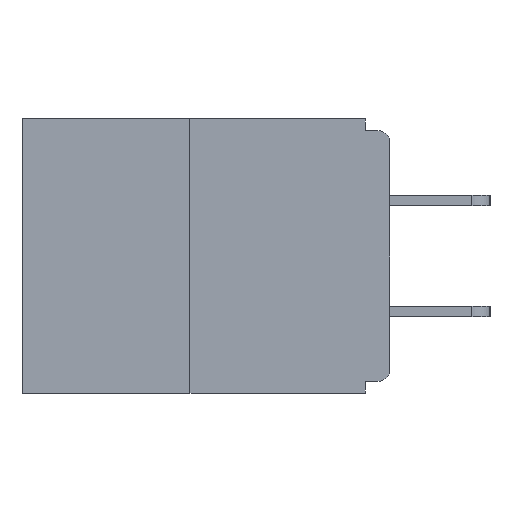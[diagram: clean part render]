
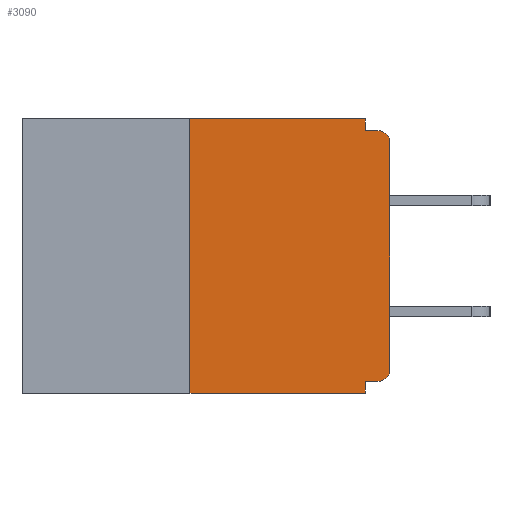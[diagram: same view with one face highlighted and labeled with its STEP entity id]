
A CAD part, left-side view. The second image highlights one B-rep face of the part: STEP entity #3090.
In plain terms, the highlighted planar face has unit normal (-1, 0, 0).
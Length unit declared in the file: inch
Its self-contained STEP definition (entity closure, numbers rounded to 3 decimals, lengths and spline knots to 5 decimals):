
#253 = DIRECTION ( 'NONE',  ( 0., 0., -1. ) ) ;
#407 = EDGE_LOOP ( 'NONE', ( #10331, #9916, #10755, #5354, #20333, #19173, #6647, #4844, #19789, #19438 ) ) ;
#422 = CARTESIAN_POINT ( 'NONE',  ( 0., 0.25, 0. ) ) ;
#709 = AXIS2_PLACEMENT_3D ( 'NONE', #9623, #9401, #14235 ) ;
#1042 = VERTEX_POINT ( 'NONE', #7243 ) ;
#1128 = DIRECTION ( 'NONE',  ( 0., 0., -1. ) ) ;
#1490 = VERTEX_POINT ( 'NONE', #20163 ) ;
#1599 = CARTESIAN_POINT ( 'NONE',  ( 0., 0.015, -0.03 ) ) ;
#1653 = CARTESIAN_POINT ( 'NONE',  ( 0., 0.015, -0.328 ) ) ;
#1782 = DIRECTION ( 'NONE',  ( -1., 0., 0. ) ) ;
#2114 = LINE ( 'NONE', #14943, #3448 ) ;
#2615 = CARTESIAN_POINT ( 'NONE',  ( 0., 0., 0. ) ) ;
#2814 = VECTOR ( 'NONE', #1128, 39.37008 ) ;
#3090 = ADVANCED_FACE ( 'NONE', ( #9512 ), #6262, .F. ) ;
#3448 = VECTOR ( 'NONE', #12514, 39.37008 ) ;
#3585 = DIRECTION ( 'NONE',  ( -1., 0., 0. ) ) ;
#4149 = CARTESIAN_POINT ( 'NONE',  ( 0., 0.031, -0.343 ) ) ;
#4844 = ORIENTED_EDGE ( 'NONE', *, *, #12302, .T. ) ;
#5054 = VERTEX_POINT ( 'NONE', #9495 ) ;
#5354 = ORIENTED_EDGE ( 'NONE', *, *, #20335, .F. ) ;
#5478 = EDGE_CURVE ( 'NONE', #9140, #5054, #14871, .T. ) ;
#5546 = VERTEX_POINT ( 'NONE', #13493 ) ;
#6262 = PLANE ( 'NONE',  #709 ) ;
#6422 = CARTESIAN_POINT ( 'NONE',  ( 0., 0.015, -0.313 ) ) ;
#6558 = LINE ( 'NONE', #6652, #14141 ) ;
#6647 = ORIENTED_EDGE ( 'NONE', *, *, #11553, .T. ) ;
#6652 = CARTESIAN_POINT ( 'NONE',  ( 0., 0., -0.015 ) ) ;
#6838 = DIRECTION ( 'NONE',  ( 0., 0., 1. ) ) ;
#7002 = DIRECTION ( 'NONE',  ( 0., 0., -1. ) ) ;
#7243 = CARTESIAN_POINT ( 'NONE',  ( 0., 0.031, -0.343 ) ) ;
#7354 = EDGE_CURVE ( 'NONE', #11797, #17008, #15986, .T. ) ;
#7400 = DIRECTION ( 'NONE',  ( 0., -1., 0. ) ) ;
#7910 = DIRECTION ( 'NONE',  ( 0., -1., 0. ) ) ;
#8236 = VECTOR ( 'NONE', #15443, 39.37008 ) ;
#8817 = CIRCLE ( 'NONE', #11506, 0.015 ) ;
#9140 = VERTEX_POINT ( 'NONE', #10795 ) ;
#9276 = VERTEX_POINT ( 'NONE', #12464 ) ;
#9401 = DIRECTION ( 'NONE',  ( 1., 0., 0. ) ) ;
#9495 = CARTESIAN_POINT ( 'NONE',  ( 0., 0.031, -0.015 ) ) ;
#9512 = FACE_OUTER_BOUND ( 'NONE', #407, .T. ) ;
#9623 = CARTESIAN_POINT ( 'NONE',  ( 0., 0.46, 0. ) ) ;
#9916 = ORIENTED_EDGE ( 'NONE', *, *, #12842, .F. ) ;
#10331 = ORIENTED_EDGE ( 'NONE', *, *, #14225, .F. ) ;
#10597 = LINE ( 'NONE', #4149, #2814 ) ;
#10755 = ORIENTED_EDGE ( 'NONE', *, *, #12438, .T. ) ;
#10795 = CARTESIAN_POINT ( 'NONE',  ( 0., 0.031, 0. ) ) ;
#10988 = VERTEX_POINT ( 'NONE', #18246 ) ;
#11324 = CARTESIAN_POINT ( 'NONE',  ( 0., 0.031, 0. ) ) ;
#11506 = AXIS2_PLACEMENT_3D ( 'NONE', #1599, #3585, #253 ) ;
#11553 = EDGE_CURVE ( 'NONE', #17008, #1490, #18943, .T. ) ;
#11704 = AXIS2_PLACEMENT_3D ( 'NONE', #6422, #1782, #12821 ) ;
#11797 = VERTEX_POINT ( 'NONE', #1653 ) ;
#12085 = VECTOR ( 'NONE', #6838, 39.37008 ) ;
#12302 = EDGE_CURVE ( 'NONE', #1490, #5546, #8817, .T. ) ;
#12314 = DIRECTION ( 'NONE',  ( 0., -1., 0. ) ) ;
#12438 = EDGE_CURVE ( 'NONE', #9276, #1042, #20027, .T. ) ;
#12464 = CARTESIAN_POINT ( 'NONE',  ( 0., 0.25, -0.343 ) ) ;
#12514 = DIRECTION ( 'NONE',  ( 0., 1., 0. ) ) ;
#12606 = VECTOR ( 'NONE', #7002, 39.37008 ) ;
#12821 = DIRECTION ( 'NONE',  ( 0., 0., -1. ) ) ;
#12842 = EDGE_CURVE ( 'NONE', #9276, #10988, #14912, .T. ) ;
#13493 = CARTESIAN_POINT ( 'NONE',  ( 0., 0.015, -0.015 ) ) ;
#14141 = VECTOR ( 'NONE', #7910, 39.37008 ) ;
#14225 = EDGE_CURVE ( 'NONE', #10988, #9140, #18895, .T. ) ;
#14235 = DIRECTION ( 'NONE',  ( 0., 0., -1. ) ) ;
#14494 = VECTOR ( 'NONE', #7400, 39.37008 ) ;
#14818 = EDGE_CURVE ( 'NONE', #5054, #5546, #6558, .T. ) ;
#14871 = LINE ( 'NONE', #11324, #12606 ) ;
#14912 = LINE ( 'NONE', #422, #12085 ) ;
#14943 = CARTESIAN_POINT ( 'NONE',  ( 0., 0., -0.328 ) ) ;
#15443 = DIRECTION ( 'NONE',  ( 0., 0., 1. ) ) ;
#15986 = CIRCLE ( 'NONE', #11704, 0.015 ) ;
#16401 = EDGE_CURVE ( 'NONE', #11797, #17117, #2114, .T. ) ;
#16889 = VECTOR ( 'NONE', #12314, 39.37008 ) ;
#17008 = VERTEX_POINT ( 'NONE', #17772 ) ;
#17117 = VERTEX_POINT ( 'NONE', #17560 ) ;
#17560 = CARTESIAN_POINT ( 'NONE',  ( 0., 0.031, -0.328 ) ) ;
#17772 = CARTESIAN_POINT ( 'NONE',  ( 0., 0., -0.313 ) ) ;
#18246 = CARTESIAN_POINT ( 'NONE',  ( 0., 0.25, 0. ) ) ;
#18438 = CARTESIAN_POINT ( 'NONE',  ( 0., 0.46, -0.343 ) ) ;
#18895 = LINE ( 'NONE', #19007, #14494 ) ;
#18943 = LINE ( 'NONE', #2615, #8236 ) ;
#19007 = CARTESIAN_POINT ( 'NONE',  ( 0., 0.46, 0. ) ) ;
#19173 = ORIENTED_EDGE ( 'NONE', *, *, #7354, .T. ) ;
#19438 = ORIENTED_EDGE ( 'NONE', *, *, #5478, .F. ) ;
#19789 = ORIENTED_EDGE ( 'NONE', *, *, #14818, .F. ) ;
#20027 = LINE ( 'NONE', #18438, #16889 ) ;
#20163 = CARTESIAN_POINT ( 'NONE',  ( 0., 0., -0.03 ) ) ;
#20333 = ORIENTED_EDGE ( 'NONE', *, *, #16401, .F. ) ;
#20335 = EDGE_CURVE ( 'NONE', #17117, #1042, #10597, .T. ) ;
